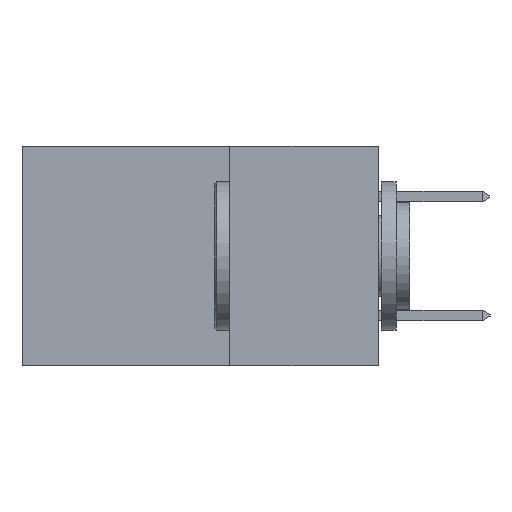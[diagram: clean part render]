
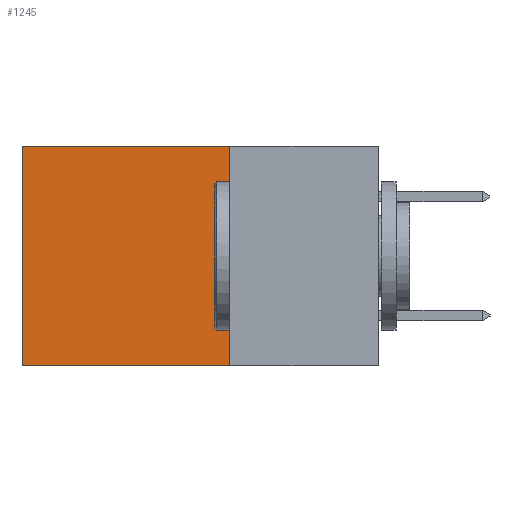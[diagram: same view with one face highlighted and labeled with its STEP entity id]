
A CAD part, left-side view. The second image highlights one B-rep face of the part: STEP entity #1245.
In plain terms, the highlighted planar face has unit normal (-1, 0, 0).
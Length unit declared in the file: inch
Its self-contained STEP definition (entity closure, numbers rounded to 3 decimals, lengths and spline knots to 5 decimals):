
#682 = PLANE ( 'NONE',  #6410 ) ;
#832 = CARTESIAN_POINT ( 'NONE',  ( 0.2615, 0.25, -0.37 ) ) ;
#861 = DIRECTION ( 'NONE',  ( 0., 0., -1. ) ) ;
#1006 = DIRECTION ( 'NONE',  ( 1., 0., 0. ) ) ;
#1041 = DIRECTION ( 'NONE',  ( 0., 0., -1. ) ) ;
#1219 = VECTOR ( 'NONE', #7237, 39.37008 ) ;
#1245 = ADVANCED_FACE ( 'NONE', ( #6733 ), #682, .F. ) ;
#1536 = DIRECTION ( 'NONE',  ( 0., 1., 0. ) ) ;
#1569 = CARTESIAN_POINT ( 'NONE',  ( 0.2615, 0.25, -0.37 ) ) ;
#1974 = EDGE_LOOP ( 'NONE', ( #5468, #11017, #6362, #12322 ) ) ;
#1989 = CARTESIAN_POINT ( 'NONE',  ( 0.2615, 0.25, -0.37 ) ) ;
#2247 = VECTOR ( 'NONE', #1536, 39.37008 ) ;
#2400 = EDGE_CURVE ( 'NONE', #7147, #11647, #8399, .T. ) ;
#2786 = VERTEX_POINT ( 'NONE', #9237 ) ;
#3230 = CARTESIAN_POINT ( 'NONE',  ( 0.2615, 0.25, 0. ) ) ;
#3772 = LINE ( 'NONE', #832, #5994 ) ;
#5468 = ORIENTED_EDGE ( 'NONE', *, *, #7869, .T. ) ;
#5976 = VECTOR ( 'NONE', #13914, 39.37008 ) ;
#5994 = VECTOR ( 'NONE', #861, 39.37008 ) ;
#6113 = CARTESIAN_POINT ( 'NONE',  ( 0.2615, 0.25, -0.37 ) ) ;
#6362 = ORIENTED_EDGE ( 'NONE', *, *, #9969, .F. ) ;
#6410 = AXIS2_PLACEMENT_3D ( 'NONE', #1989, #1006, #1041 ) ;
#6733 = FACE_OUTER_BOUND ( 'NONE', #1974, .T. ) ;
#6938 = CARTESIAN_POINT ( 'NONE',  ( 0.2615, 0.6, -0.37 ) ) ;
#7075 = LINE ( 'NONE', #6938, #1219 ) ;
#7147 = VERTEX_POINT ( 'NONE', #6113 ) ;
#7237 = DIRECTION ( 'NONE',  ( 0., 0., -1. ) ) ;
#7869 = EDGE_CURVE ( 'NONE', #2786, #11647, #7075, .T. ) ;
#8190 = VERTEX_POINT ( 'NONE', #3230 ) ;
#8399 = LINE ( 'NONE', #1569, #2247 ) ;
#8729 = CARTESIAN_POINT ( 'NONE',  ( 0.2615, 0.6, -0.37 ) ) ;
#8842 = LINE ( 'NONE', #11916, #5976 ) ;
#9237 = CARTESIAN_POINT ( 'NONE',  ( 0.2615, 0.6, 0. ) ) ;
#9969 = EDGE_CURVE ( 'NONE', #8190, #7147, #3772, .T. ) ;
#11017 = ORIENTED_EDGE ( 'NONE', *, *, #2400, .F. ) ;
#11647 = VERTEX_POINT ( 'NONE', #8729 ) ;
#11711 = EDGE_CURVE ( 'NONE', #8190, #2786, #8842, .T. ) ;
#11916 = CARTESIAN_POINT ( 'NONE',  ( 0.2615, 0.25, 0. ) ) ;
#12322 = ORIENTED_EDGE ( 'NONE', *, *, #11711, .T. ) ;
#13914 = DIRECTION ( 'NONE',  ( 0., 1., 0. ) ) ;
